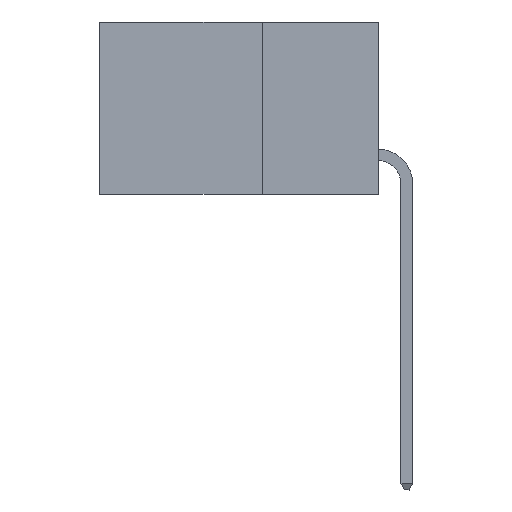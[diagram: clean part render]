
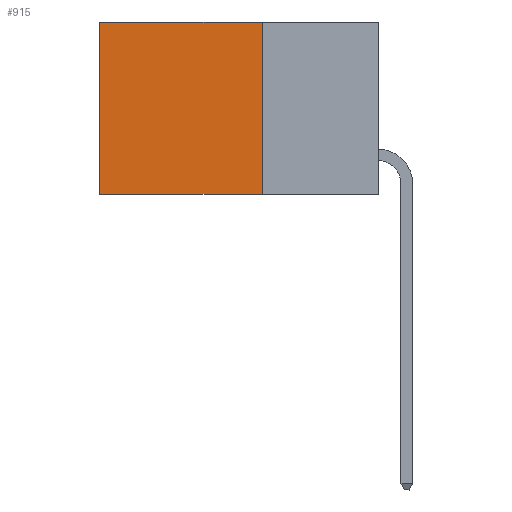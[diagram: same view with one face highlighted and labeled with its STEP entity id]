
A CAD part, left-side view. The second image highlights one B-rep face of the part: STEP entity #915.
In plain terms, the highlighted planar face has unit normal (-1, 0, 0).
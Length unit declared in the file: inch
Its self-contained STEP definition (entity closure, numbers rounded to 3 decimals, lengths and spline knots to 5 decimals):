
#500 = VECTOR ( 'NONE', #7955, 39.37008 ) ;
#595 = EDGE_CURVE ( 'NONE', #6383, #8181, #4308, .T. ) ;
#754 = FACE_OUTER_BOUND ( 'NONE', #2325, .T. ) ;
#915 = ADVANCED_FACE ( 'NONE', ( #754 ), #2802, .F. ) ;
#1234 = ORIENTED_EDGE ( 'NONE', *, *, #2097, .T. ) ;
#1303 = CARTESIAN_POINT ( 'NONE',  ( 0.2615, 0.25, 0. ) ) ;
#1380 = ORIENTED_EDGE ( 'NONE', *, *, #3108, .F. ) ;
#1408 = AXIS2_PLACEMENT_3D ( 'NONE', #3664, #7736, #2223 ) ;
#2097 = EDGE_CURVE ( 'NONE', #6744, #5000, #5373, .T. ) ;
#2204 = EDGE_CURVE ( 'NONE', #5000, #8181, #5390, .T. ) ;
#2223 = DIRECTION ( 'NONE',  ( 0., 0., -1. ) ) ;
#2325 = EDGE_LOOP ( 'NONE', ( #3211, #7532, #1380, #1234 ) ) ;
#2358 = VECTOR ( 'NONE', #8196, 39.37008 ) ;
#2594 = CARTESIAN_POINT ( 'NONE',  ( 0.2615, 0.25, 0. ) ) ;
#2802 = PLANE ( 'NONE',  #1408 ) ;
#3108 = EDGE_CURVE ( 'NONE', #6744, #6383, #7266, .T. ) ;
#3135 = CARTESIAN_POINT ( 'NONE',  ( 0.2615, 0.25, -0.37 ) ) ;
#3211 = ORIENTED_EDGE ( 'NONE', *, *, #2204, .T. ) ;
#3664 = CARTESIAN_POINT ( 'NONE',  ( 0.2615, 0.25, -0.37 ) ) ;
#4144 = CARTESIAN_POINT ( 'NONE',  ( 0.2615, 0.6, 0. ) ) ;
#4220 = DIRECTION ( 'NONE',  ( 0., 1., 0. ) ) ;
#4308 = LINE ( 'NONE', #7111, #7752 ) ;
#4478 = CARTESIAN_POINT ( 'NONE',  ( 0.2615, 0.25, -0.37 ) ) ;
#4816 = VECTOR ( 'NONE', #6094, 39.37008 ) ;
#5000 = VERTEX_POINT ( 'NONE', #4144 ) ;
#5373 = LINE ( 'NONE', #2594, #4816 ) ;
#5390 = LINE ( 'NONE', #7240, #500 ) ;
#6094 = DIRECTION ( 'NONE',  ( 0., 1., 0. ) ) ;
#6383 = VERTEX_POINT ( 'NONE', #4478 ) ;
#6744 = VERTEX_POINT ( 'NONE', #1303 ) ;
#7111 = CARTESIAN_POINT ( 'NONE',  ( 0.2615, 0.25, -0.37 ) ) ;
#7240 = CARTESIAN_POINT ( 'NONE',  ( 0.2615, 0.6, -0.37 ) ) ;
#7266 = LINE ( 'NONE', #3135, #2358 ) ;
#7532 = ORIENTED_EDGE ( 'NONE', *, *, #595, .F. ) ;
#7736 = DIRECTION ( 'NONE',  ( 1., 0., 0. ) ) ;
#7752 = VECTOR ( 'NONE', #4220, 39.37008 ) ;
#7955 = DIRECTION ( 'NONE',  ( 0., 0., -1. ) ) ;
#8181 = VERTEX_POINT ( 'NONE', #8585 ) ;
#8196 = DIRECTION ( 'NONE',  ( 0., 0., -1. ) ) ;
#8585 = CARTESIAN_POINT ( 'NONE',  ( 0.2615, 0.6, -0.37 ) ) ;
